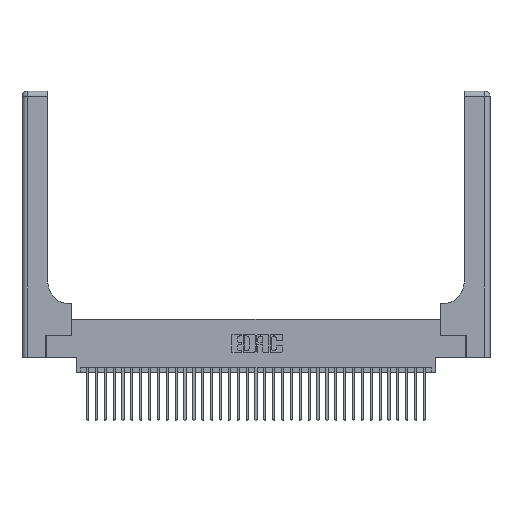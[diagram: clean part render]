
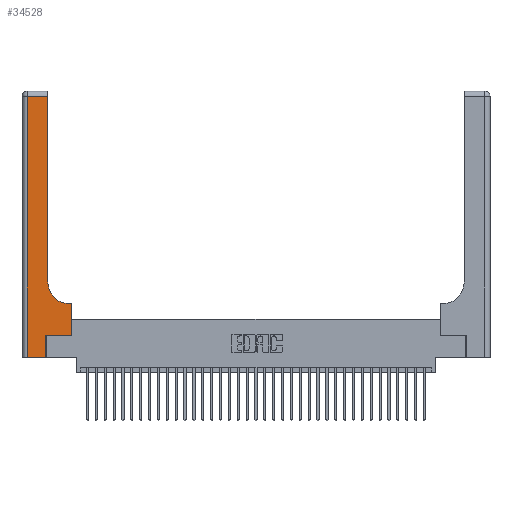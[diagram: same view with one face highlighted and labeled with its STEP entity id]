
A CAD part, top view. The second image highlights one B-rep face of the part: STEP entity #34528.
In plain terms, the highlighted planar face has unit normal (0, 0, 1).
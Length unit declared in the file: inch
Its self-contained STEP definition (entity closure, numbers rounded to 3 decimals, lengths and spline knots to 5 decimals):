
#152 = VECTOR ( 'NONE', #30045, 39.37008 ) ;
#430 = DIRECTION ( 'NONE',  ( 1., 0., 0. ) ) ;
#546 = CARTESIAN_POINT ( 'NONE',  ( 0.5585, 0.25, 0.37 ) ) ;
#2024 = EDGE_CURVE ( 'NONE', #11062, #35676, #9871, .T. ) ;
#2382 = LINE ( 'NONE', #17658, #30547 ) ;
#3254 = CARTESIAN_POINT ( 'NONE',  ( 0.5415, 0.85, 0.37 ) ) ;
#3500 = EDGE_CURVE ( 'NONE', #34876, #11062, #2382, .T. ) ;
#4509 = DIRECTION ( 'NONE',  ( 0., -1., 0. ) ) ;
#4817 = CARTESIAN_POINT ( 'NONE',  ( 0.2915, 0.6, 0.37 ) ) ;
#5322 = LINE ( 'NONE', #13575, #12819 ) ;
#5477 = EDGE_CURVE ( 'NONE', #26472, #16013, #33229, .T. ) ;
#5736 = DIRECTION ( 'NONE',  ( 0., 1., 0. ) ) ;
#5974 = DIRECTION ( 'NONE',  ( 0., 1., 0. ) ) ;
#6352 = VECTOR ( 'NONE', #33389, 39.37008 ) ;
#7100 = CARTESIAN_POINT ( 'NONE',  ( 0.06, 3., 0.37 ) ) ;
#7659 = EDGE_LOOP ( 'NONE', ( #30750, #10821, #16101, #23728, #32484, #36055, #9191, #35778, #14537 ) ) ;
#7949 = LINE ( 'NONE', #25686, #34236 ) ;
#8147 = VERTEX_POINT ( 'NONE', #22497 ) ;
#9191 = ORIENTED_EDGE ( 'NONE', *, *, #15243, .T. ) ;
#9569 = VECTOR ( 'NONE', #16440, 39.37008 ) ;
#9789 = FACE_OUTER_BOUND ( 'NONE', #7659, .T. ) ;
#9871 = LINE ( 'NONE', #7100, #12541 ) ;
#10821 = ORIENTED_EDGE ( 'NONE', *, *, #3500, .T. ) ;
#10955 = AXIS2_PLACEMENT_3D ( 'NONE', #3254, #25665, #430 ) ;
#10998 = EDGE_CURVE ( 'NONE', #26819, #33174, #21929, .T. ) ;
#11062 = VERTEX_POINT ( 'NONE', #17484 ) ;
#12082 = DIRECTION ( 'NONE',  ( 1., 0., 0. ) ) ;
#12156 = CARTESIAN_POINT ( 'NONE',  ( 0.269, 0.25, 0.37 ) ) ;
#12541 = VECTOR ( 'NONE', #4509, 39.37008 ) ;
#12773 = CIRCLE ( 'NONE', #10955, 0.25 ) ;
#12819 = VECTOR ( 'NONE', #5974, 39.37008 ) ;
#13575 = CARTESIAN_POINT ( 'NONE',  ( 0.5585, 0.25, 0.37 ) ) ;
#13804 = EDGE_CURVE ( 'NONE', #8147, #34876, #29116, .T. ) ;
#14537 = ORIENTED_EDGE ( 'NONE', *, *, #36333, .T. ) ;
#15243 = EDGE_CURVE ( 'NONE', #16013, #26819, #5322, .T. ) ;
#16013 = VERTEX_POINT ( 'NONE', #546 ) ;
#16101 = ORIENTED_EDGE ( 'NONE', *, *, #2024, .T. ) ;
#16440 = DIRECTION ( 'NONE',  ( -1., 0., 0. ) ) ;
#17178 = CARTESIAN_POINT ( 'NONE',  ( 0., 3., 0.37 ) ) ;
#17464 = AXIS2_PLACEMENT_3D ( 'NONE', #17178, #33861, #34313 ) ;
#17484 = CARTESIAN_POINT ( 'NONE',  ( 0.06, 2.94, 0.37 ) ) ;
#17658 = CARTESIAN_POINT ( 'NONE',  ( 0., 2.94, 0.37 ) ) ;
#20568 = EDGE_CURVE ( 'NONE', #35676, #33355, #23199, .T. ) ;
#21929 = LINE ( 'NONE', #4817, #9569 ) ;
#22497 = CARTESIAN_POINT ( 'NONE',  ( 0.2915, 0.85, 0.37 ) ) ;
#23199 = LINE ( 'NONE', #31933, #32429 ) ;
#23728 = ORIENTED_EDGE ( 'NONE', *, *, #20568, .T. ) ;
#24653 = CARTESIAN_POINT ( 'NONE',  ( 0.2915, 3., 0.37 ) ) ;
#25665 = DIRECTION ( 'NONE',  ( 0., 0., -1. ) ) ;
#25686 = CARTESIAN_POINT ( 'NONE',  ( 0.269, 0., 0.37 ) ) ;
#26276 = CARTESIAN_POINT ( 'NONE',  ( 0.269, 0.25, 0.37 ) ) ;
#26472 = VERTEX_POINT ( 'NONE', #12156 ) ;
#26819 = VERTEX_POINT ( 'NONE', #27765 ) ;
#26992 = CARTESIAN_POINT ( 'NONE',  ( 0.2915, 2.94, 0.37 ) ) ;
#27765 = CARTESIAN_POINT ( 'NONE',  ( 0.5585, 0.6, 0.37 ) ) ;
#28243 = EDGE_CURVE ( 'NONE', #33355, #26472, #7949, .T. ) ;
#28259 = CARTESIAN_POINT ( 'NONE',  ( 0.269, 0., 0.37 ) ) ;
#29116 = LINE ( 'NONE', #24653, #152 ) ;
#29207 = DIRECTION ( 'NONE',  ( -1., 0., 0. ) ) ;
#30045 = DIRECTION ( 'NONE',  ( 0., 1., 0. ) ) ;
#30124 = CARTESIAN_POINT ( 'NONE',  ( 0.5415, 0.6, 0.37 ) ) ;
#30401 = CARTESIAN_POINT ( 'NONE',  ( 0.06, 0., 0.37 ) ) ;
#30547 = VECTOR ( 'NONE', #29207, 39.37008 ) ;
#30750 = ORIENTED_EDGE ( 'NONE', *, *, #13804, .T. ) ;
#31933 = CARTESIAN_POINT ( 'NONE',  ( 0., 0., 0.37 ) ) ;
#32429 = VECTOR ( 'NONE', #12082, 39.37008 ) ;
#32484 = ORIENTED_EDGE ( 'NONE', *, *, #28243, .T. ) ;
#33174 = VERTEX_POINT ( 'NONE', #30124 ) ;
#33229 = LINE ( 'NONE', #26276, #6352 ) ;
#33355 = VERTEX_POINT ( 'NONE', #28259 ) ;
#33389 = DIRECTION ( 'NONE',  ( 1., 0., 0. ) ) ;
#33861 = DIRECTION ( 'NONE',  ( 0., 0., -1. ) ) ;
#33980 = PLANE ( 'NONE',  #17464 ) ;
#34236 = VECTOR ( 'NONE', #5736, 39.37008 ) ;
#34313 = DIRECTION ( 'NONE',  ( -1., 0., 0. ) ) ;
#34528 = ADVANCED_FACE ( 'NONE', ( #9789 ), #33980, .F. ) ;
#34876 = VERTEX_POINT ( 'NONE', #26992 ) ;
#35676 = VERTEX_POINT ( 'NONE', #30401 ) ;
#35778 = ORIENTED_EDGE ( 'NONE', *, *, #10998, .T. ) ;
#36055 = ORIENTED_EDGE ( 'NONE', *, *, #5477, .T. ) ;
#36333 = EDGE_CURVE ( 'NONE', #33174, #8147, #12773, .T. ) ;
